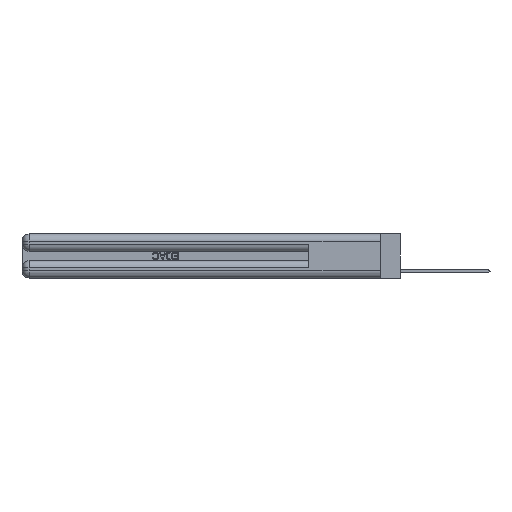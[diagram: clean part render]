
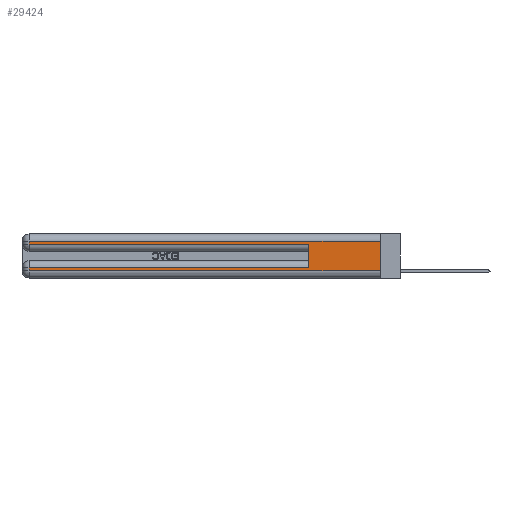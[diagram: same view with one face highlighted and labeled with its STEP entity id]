
A CAD part, left-side view. The second image highlights one B-rep face of the part: STEP entity #29424.
In plain terms, the highlighted planar face has unit normal (-1, 0, 0).
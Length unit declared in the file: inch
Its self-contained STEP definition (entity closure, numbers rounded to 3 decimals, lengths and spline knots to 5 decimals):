
#207 = EDGE_LOOP ( 'NONE', ( #22917, #5267, #29301, #1763, #15778, #13786, #25110, #30226 ) ) ;
#1190 = LINE ( 'NONE', #29893, #13843 ) ;
#1244 = EDGE_CURVE ( 'NONE', #24923, #26997, #22632, .T. ) ;
#1373 = DIRECTION ( 'NONE',  ( 0., 1., 0. ) ) ;
#1763 = ORIENTED_EDGE ( 'NONE', *, *, #1244, .T. ) ;
#2007 = EDGE_CURVE ( 'NONE', #18736, #24923, #20049, .T. ) ;
#4454 = VERTEX_POINT ( 'NONE', #25791 ) ;
#4813 = CARTESIAN_POINT ( 'NONE',  ( 0., 0.6, 0.085 ) ) ;
#4901 = VERTEX_POINT ( 'NONE', #22923 ) ;
#5267 = ORIENTED_EDGE ( 'NONE', *, *, #9374, .T. ) ;
#5418 = AXIS2_PLACEMENT_3D ( 'NONE', #13307, #10928, #11398 ) ;
#5630 = VECTOR ( 'NONE', #16818, 39.37008 ) ;
#5973 = CARTESIAN_POINT ( 'NONE',  ( 0., 0., 0.285 ) ) ;
#6459 = CARTESIAN_POINT ( 'NONE',  ( 0., 0., 0.31 ) ) ;
#6755 = VECTOR ( 'NONE', #10107, 39.37008 ) ;
#7197 = VECTOR ( 'NONE', #22911, 39.37008 ) ;
#7286 = CARTESIAN_POINT ( 'NONE',  ( 0., 2.94, 0.37 ) ) ;
#7942 = VERTEX_POINT ( 'NONE', #4813 ) ;
#8212 = LINE ( 'NONE', #6459, #27039 ) ;
#9234 = EDGE_CURVE ( 'NONE', #4901, #22191, #17899, .T. ) ;
#9374 = EDGE_CURVE ( 'NONE', #4454, #18736, #8212, .T. ) ;
#9571 = LINE ( 'NONE', #21637, #26430 ) ;
#10107 = DIRECTION ( 'NONE',  ( 0., -1., 0. ) ) ;
#10418 = VERTEX_POINT ( 'NONE', #19491 ) ;
#10430 = EDGE_CURVE ( 'NONE', #10418, #4901, #22030, .T. ) ;
#10906 = DIRECTION ( 'NONE',  ( 0., -1., 0. ) ) ;
#10928 = DIRECTION ( 'NONE',  ( 1., 0., 0. ) ) ;
#10986 = EDGE_CURVE ( 'NONE', #4454, #22191, #17867, .T. ) ;
#11398 = DIRECTION ( 'NONE',  ( 0., 0., -1. ) ) ;
#12921 = CARTESIAN_POINT ( 'NONE',  ( 0., 0., 0.37 ) ) ;
#13307 = CARTESIAN_POINT ( 'NONE',  ( 0., 0., 0.37 ) ) ;
#13785 = FACE_OUTER_BOUND ( 'NONE', #207, .T. ) ;
#13786 = ORIENTED_EDGE ( 'NONE', *, *, #21336, .T. ) ;
#13843 = VECTOR ( 'NONE', #30059, 39.37008 ) ;
#14755 = VECTOR ( 'NONE', #10906, 39.37008 ) ;
#14998 = DIRECTION ( 'NONE',  ( 0., 0., -1. ) ) ;
#15221 = VECTOR ( 'NONE', #14998, 39.37008 ) ;
#15778 = ORIENTED_EDGE ( 'NONE', *, *, #22098, .F. ) ;
#16682 = CARTESIAN_POINT ( 'NONE',  ( 0., 2.94, 0.285 ) ) ;
#16818 = DIRECTION ( 'NONE',  ( 0., 0., -1. ) ) ;
#17867 = LINE ( 'NONE', #12921, #15221 ) ;
#17899 = LINE ( 'NONE', #27222, #6755 ) ;
#18725 = CARTESIAN_POINT ( 'NONE',  ( 0., 2.94, 0.31 ) ) ;
#18736 = VERTEX_POINT ( 'NONE', #18725 ) ;
#19491 = CARTESIAN_POINT ( 'NONE',  ( 0., 2.94, 0.085 ) ) ;
#20049 = LINE ( 'NONE', #27651, #7197 ) ;
#21336 = EDGE_CURVE ( 'NONE', #7942, #10418, #9571, .T. ) ;
#21637 = CARTESIAN_POINT ( 'NONE',  ( 0., 0., 0.085 ) ) ;
#22030 = LINE ( 'NONE', #7286, #5630 ) ;
#22098 = EDGE_CURVE ( 'NONE', #7942, #26997, #1190, .T. ) ;
#22191 = VERTEX_POINT ( 'NONE', #30688 ) ;
#22632 = LINE ( 'NONE', #5973, #14755 ) ;
#22911 = DIRECTION ( 'NONE',  ( 0., 0., -1. ) ) ;
#22917 = ORIENTED_EDGE ( 'NONE', *, *, #10986, .F. ) ;
#22923 = CARTESIAN_POINT ( 'NONE',  ( 0., 2.94, 0.06 ) ) ;
#23461 = PLANE ( 'NONE',  #5418 ) ;
#24923 = VERTEX_POINT ( 'NONE', #16682 ) ;
#25110 = ORIENTED_EDGE ( 'NONE', *, *, #10430, .T. ) ;
#25791 = CARTESIAN_POINT ( 'NONE',  ( 0., 0., 0.31 ) ) ;
#26257 = CARTESIAN_POINT ( 'NONE',  ( 0., 0.6, 0.285 ) ) ;
#26430 = VECTOR ( 'NONE', #31285, 39.37008 ) ;
#26997 = VERTEX_POINT ( 'NONE', #26257 ) ;
#27039 = VECTOR ( 'NONE', #1373, 39.37008 ) ;
#27222 = CARTESIAN_POINT ( 'NONE',  ( 0., 0., 0.06 ) ) ;
#27651 = CARTESIAN_POINT ( 'NONE',  ( 0., 2.94, 0.37 ) ) ;
#29301 = ORIENTED_EDGE ( 'NONE', *, *, #2007, .T. ) ;
#29424 = ADVANCED_FACE ( 'NONE', ( #13785 ), #23461, .F. ) ;
#29893 = CARTESIAN_POINT ( 'NONE',  ( 0., 0.6, 0.145 ) ) ;
#30059 = DIRECTION ( 'NONE',  ( 0., 0., 1. ) ) ;
#30226 = ORIENTED_EDGE ( 'NONE', *, *, #9234, .T. ) ;
#30688 = CARTESIAN_POINT ( 'NONE',  ( 0., 0., 0.06 ) ) ;
#31285 = DIRECTION ( 'NONE',  ( 0., 1., 0. ) ) ;
